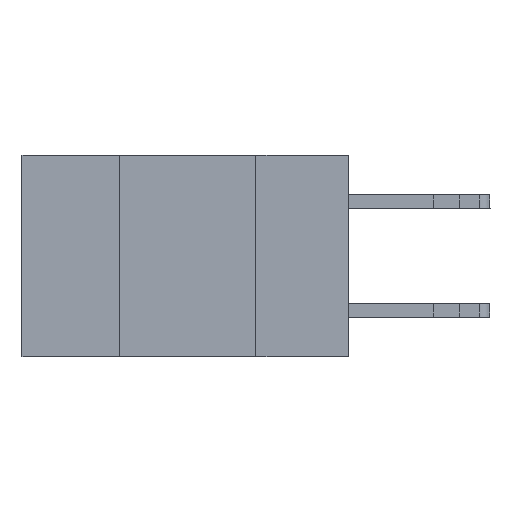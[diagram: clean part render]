
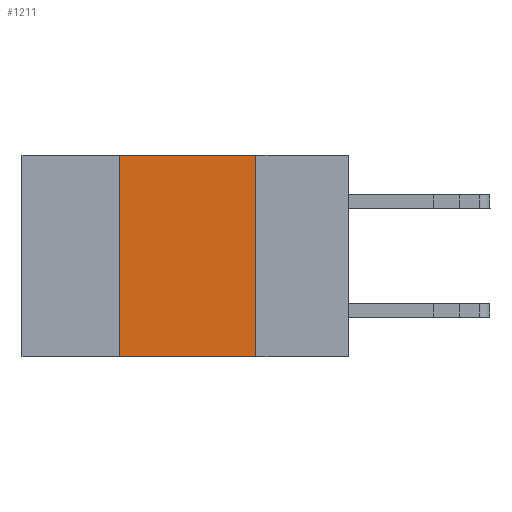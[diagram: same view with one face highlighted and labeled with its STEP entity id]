
A CAD part, left-side view. The second image highlights one B-rep face of the part: STEP entity #1211.
In plain terms, the highlighted planar face has unit normal (-1, 0, 0).
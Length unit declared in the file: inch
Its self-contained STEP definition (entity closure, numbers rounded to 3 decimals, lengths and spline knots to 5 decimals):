
#114 = ORIENTED_EDGE ( 'NONE', *, *, #6166, .F. ) ;
#1073 = DIRECTION ( 'NONE',  ( 0., -1., 0. ) ) ;
#1197 = VERTEX_POINT ( 'NONE', #7287 ) ;
#1211 = ADVANCED_FACE ( 'NONE', ( #6370 ), #2914, .F. ) ;
#1417 = VECTOR ( 'NONE', #9985, 39.37008 ) ;
#1720 = CARTESIAN_POINT ( 'NONE',  ( 0., 0.6, -0.37 ) ) ;
#1771 = DIRECTION ( 'NONE',  ( 1., 0., 0. ) ) ;
#2794 = LINE ( 'NONE', #8944, #7579 ) ;
#2914 = PLANE ( 'NONE',  #7480 ) ;
#4823 = VECTOR ( 'NONE', #10127, 39.37008 ) ;
#5272 = CARTESIAN_POINT ( 'NONE',  ( 0., 0.42, 0. ) ) ;
#5289 = EDGE_CURVE ( 'NONE', #6585, #7780, #6946, .T. ) ;
#5382 = EDGE_LOOP ( 'NONE', ( #8442, #10529, #114, #7594 ) ) ;
#5447 = EDGE_CURVE ( 'NONE', #5922, #1197, #2794, .T. ) ;
#5922 = VERTEX_POINT ( 'NONE', #5272 ) ;
#5976 = DIRECTION ( 'NONE',  ( 0., -1., 0. ) ) ;
#6166 = EDGE_CURVE ( 'NONE', #6585, #5922, #7605, .T. ) ;
#6370 = FACE_OUTER_BOUND ( 'NONE', #5382, .T. ) ;
#6500 = CARTESIAN_POINT ( 'NONE',  ( 0., 0.17, -0.37 ) ) ;
#6585 = VERTEX_POINT ( 'NONE', #10963 ) ;
#6946 = LINE ( 'NONE', #1720, #7931 ) ;
#7287 = CARTESIAN_POINT ( 'NONE',  ( 0., 0.17, 0. ) ) ;
#7467 = LINE ( 'NONE', #6500, #1417 ) ;
#7480 = AXIS2_PLACEMENT_3D ( 'NONE', #9624, #1771, #7965 ) ;
#7579 = VECTOR ( 'NONE', #1073, 39.37008 ) ;
#7594 = ORIENTED_EDGE ( 'NONE', *, *, #5289, .T. ) ;
#7605 = LINE ( 'NONE', #9435, #4823 ) ;
#7780 = VERTEX_POINT ( 'NONE', #9370 ) ;
#7931 = VECTOR ( 'NONE', #5976, 39.37008 ) ;
#7965 = DIRECTION ( 'NONE',  ( 0., 0., -1. ) ) ;
#8442 = ORIENTED_EDGE ( 'NONE', *, *, #11306, .F. ) ;
#8944 = CARTESIAN_POINT ( 'NONE',  ( 0., 0.6, 0. ) ) ;
#9370 = CARTESIAN_POINT ( 'NONE',  ( 0., 0.17, -0.37 ) ) ;
#9435 = CARTESIAN_POINT ( 'NONE',  ( 0., 0.42, -0.37 ) ) ;
#9624 = CARTESIAN_POINT ( 'NONE',  ( 0., 0.6, 0. ) ) ;
#9985 = DIRECTION ( 'NONE',  ( 0., 0., -1. ) ) ;
#10127 = DIRECTION ( 'NONE',  ( 0., 0., 1. ) ) ;
#10529 = ORIENTED_EDGE ( 'NONE', *, *, #5447, .F. ) ;
#10963 = CARTESIAN_POINT ( 'NONE',  ( 0., 0.42, -0.37 ) ) ;
#11306 = EDGE_CURVE ( 'NONE', #1197, #7780, #7467, .T. ) ;
